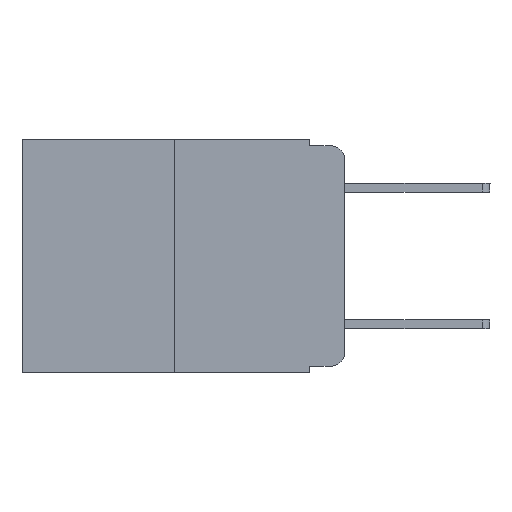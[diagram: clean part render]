
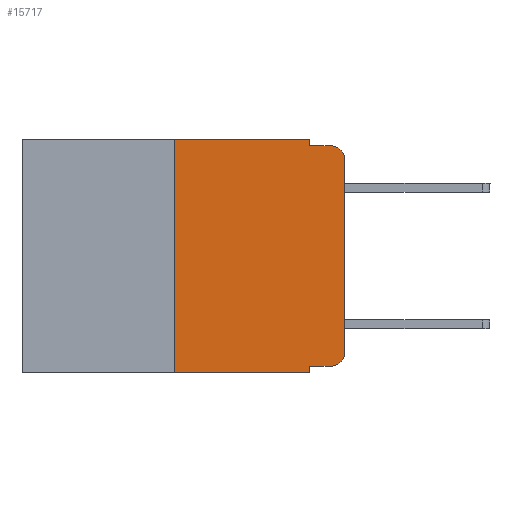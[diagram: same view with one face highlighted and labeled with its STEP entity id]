
A CAD part, left-side view. The second image highlights one B-rep face of the part: STEP entity #15717.
In plain terms, the highlighted planar face has unit normal (-1, 0, 0).
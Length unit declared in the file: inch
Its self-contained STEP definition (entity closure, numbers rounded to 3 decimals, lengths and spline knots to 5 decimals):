
#430 = VERTEX_POINT ( 'NONE', #24425 ) ;
#989 = VECTOR ( 'NONE', #17056, 39.37008 ) ;
#1262 = LINE ( 'NONE', #10954, #9481 ) ;
#1275 = DIRECTION ( 'NONE',  ( 0., -1., 0. ) ) ;
#1379 = CARTESIAN_POINT ( 'NONE',  ( 0., 0.051, 0. ) ) ;
#2024 = CARTESIAN_POINT ( 'NONE',  ( 0., 0.051, -0.343 ) ) ;
#2094 = CARTESIAN_POINT ( 'NONE',  ( 0., 0.051, 0. ) ) ;
#2212 = CIRCLE ( 'NONE', #17054, 0.02 ) ;
#2720 = VERTEX_POINT ( 'NONE', #14992 ) ;
#2901 = CARTESIAN_POINT ( 'NONE',  ( 0., 0.051, 0. ) ) ;
#2908 = CARTESIAN_POINT ( 'NONE',  ( 0., 0.051, -0.333 ) ) ;
#2981 = VERTEX_POINT ( 'NONE', #8817 ) ;
#3386 = ORIENTED_EDGE ( 'NONE', *, *, #4770, .F. ) ;
#3758 = CARTESIAN_POINT ( 'NONE',  ( 0., 0.473, 0. ) ) ;
#4460 = LINE ( 'NONE', #10531, #989 ) ;
#4770 = EDGE_CURVE ( 'NONE', #16904, #23229, #1262, .T. ) ;
#5039 = DIRECTION ( 'NONE',  ( 0., -1., 0. ) ) ;
#5089 = ORIENTED_EDGE ( 'NONE', *, *, #16023, .T. ) ;
#5216 = EDGE_CURVE ( 'NONE', #25770, #17007, #4460, .T. ) ;
#5581 = DIRECTION ( 'NONE',  ( 0., 0., 1. ) ) ;
#5851 = DIRECTION ( 'NONE',  ( -1., 0., 0. ) ) ;
#5925 = ORIENTED_EDGE ( 'NONE', *, *, #24946, .T. ) ;
#6001 = EDGE_CURVE ( 'NONE', #18754, #6671, #21037, .T. ) ;
#6176 = ORIENTED_EDGE ( 'NONE', *, *, #22233, .F. ) ;
#6227 = DIRECTION ( 'NONE',  ( 1., 0., 0. ) ) ;
#6426 = CARTESIAN_POINT ( 'NONE',  ( 0., 0.473, 0. ) ) ;
#6446 = ORIENTED_EDGE ( 'NONE', *, *, #5216, .T. ) ;
#6671 = VERTEX_POINT ( 'NONE', #2024 ) ;
#7207 = EDGE_CURVE ( 'NONE', #17007, #23229, #19730, .T. ) ;
#7561 = CARTESIAN_POINT ( 'NONE',  ( 0., 0.02, -0.313 ) ) ;
#7942 = VECTOR ( 'NONE', #9463, 39.37008 ) ;
#8163 = ORIENTED_EDGE ( 'NONE', *, *, #21333, .F. ) ;
#8817 = CARTESIAN_POINT ( 'NONE',  ( 0., 0.02, -0.333 ) ) ;
#9109 = AXIS2_PLACEMENT_3D ( 'NONE', #13552, #14403, #20532 ) ;
#9279 = LINE ( 'NONE', #25662, #22911 ) ;
#9463 = DIRECTION ( 'NONE',  ( 0., 0., -1. ) ) ;
#9481 = VECTOR ( 'NONE', #14818, 39.37008 ) ;
#9502 = LINE ( 'NONE', #25603, #10619 ) ;
#9643 = EDGE_CURVE ( 'NONE', #430, #2720, #9279, .T. ) ;
#10252 = VERTEX_POINT ( 'NONE', #2094 ) ;
#10531 = CARTESIAN_POINT ( 'NONE',  ( 0., 0., 0. ) ) ;
#10619 = VECTOR ( 'NONE', #1275, 39.37008 ) ;
#10954 = CARTESIAN_POINT ( 'NONE',  ( 0., 0.051, -0.01 ) ) ;
#11247 = VECTOR ( 'NONE', #16928, 39.37008 ) ;
#11911 = ORIENTED_EDGE ( 'NONE', *, *, #7207, .T. ) ;
#12222 = PLANE ( 'NONE',  #22515 ) ;
#13433 = LINE ( 'NONE', #25638, #14029 ) ;
#13552 = CARTESIAN_POINT ( 'NONE',  ( 0., 0.02, -0.03 ) ) ;
#13570 = CARTESIAN_POINT ( 'NONE',  ( 0., 0.051, -0.01 ) ) ;
#13941 = DIRECTION ( 'NONE',  ( 0., 0., -1. ) ) ;
#14029 = VECTOR ( 'NONE', #5039, 39.37008 ) ;
#14403 = DIRECTION ( 'NONE',  ( -1., 0., 0. ) ) ;
#14818 = DIRECTION ( 'NONE',  ( 0., -1., 0. ) ) ;
#14992 = CARTESIAN_POINT ( 'NONE',  ( 0., 0.25, 0. ) ) ;
#15717 = ADVANCED_FACE ( 'NONE', ( #24451 ), #12222, .F. ) ;
#15843 = ORIENTED_EDGE ( 'NONE', *, *, #6001, .F. ) ;
#15868 = CARTESIAN_POINT ( 'NONE',  ( 0., 0., -0.313 ) ) ;
#16023 = EDGE_CURVE ( 'NONE', #430, #6671, #13433, .T. ) ;
#16904 = VERTEX_POINT ( 'NONE', #13570 ) ;
#16928 = DIRECTION ( 'NONE',  ( 0., -1., 0. ) ) ;
#17007 = VERTEX_POINT ( 'NONE', #21934 ) ;
#17054 = AXIS2_PLACEMENT_3D ( 'NONE', #7561, #5851, #13941 ) ;
#17056 = DIRECTION ( 'NONE',  ( 0., 0., 1. ) ) ;
#17071 = LINE ( 'NONE', #6426, #11247 ) ;
#17943 = DIRECTION ( 'NONE',  ( 0., 0., -1. ) ) ;
#18687 = DIRECTION ( 'NONE',  ( 0., 0., -1. ) ) ;
#18754 = VERTEX_POINT ( 'NONE', #2908 ) ;
#19730 = CIRCLE ( 'NONE', #9109, 0.02 ) ;
#20532 = DIRECTION ( 'NONE',  ( 0., 0., -1. ) ) ;
#21037 = LINE ( 'NONE', #1379, #7942 ) ;
#21082 = LINE ( 'NONE', #2901, #22082 ) ;
#21333 = EDGE_CURVE ( 'NONE', #2720, #10252, #17071, .T. ) ;
#21934 = CARTESIAN_POINT ( 'NONE',  ( 0., 0., -0.03 ) ) ;
#22082 = VECTOR ( 'NONE', #18687, 39.37008 ) ;
#22233 = EDGE_CURVE ( 'NONE', #10252, #16904, #21082, .T. ) ;
#22515 = AXIS2_PLACEMENT_3D ( 'NONE', #3758, #6227, #17943 ) ;
#22911 = VECTOR ( 'NONE', #5581, 39.37008 ) ;
#23229 = VERTEX_POINT ( 'NONE', #25682 ) ;
#23940 = EDGE_CURVE ( 'NONE', #18754, #2981, #9502, .T. ) ;
#24425 = CARTESIAN_POINT ( 'NONE',  ( 0., 0.25, -0.343 ) ) ;
#24451 = FACE_OUTER_BOUND ( 'NONE', #26135, .T. ) ;
#24946 = EDGE_CURVE ( 'NONE', #2981, #25770, #2212, .T. ) ;
#25289 = ORIENTED_EDGE ( 'NONE', *, *, #9643, .F. ) ;
#25603 = CARTESIAN_POINT ( 'NONE',  ( 0., 0.051, -0.333 ) ) ;
#25638 = CARTESIAN_POINT ( 'NONE',  ( 0., 0.473, -0.343 ) ) ;
#25662 = CARTESIAN_POINT ( 'NONE',  ( 0., 0.25, 0. ) ) ;
#25682 = CARTESIAN_POINT ( 'NONE',  ( 0., 0.02, -0.01 ) ) ;
#25770 = VERTEX_POINT ( 'NONE', #15868 ) ;
#26067 = ORIENTED_EDGE ( 'NONE', *, *, #23940, .T. ) ;
#26135 = EDGE_LOOP ( 'NONE', ( #6446, #11911, #3386, #6176, #8163, #25289, #5089, #15843, #26067, #5925 ) ) ;
